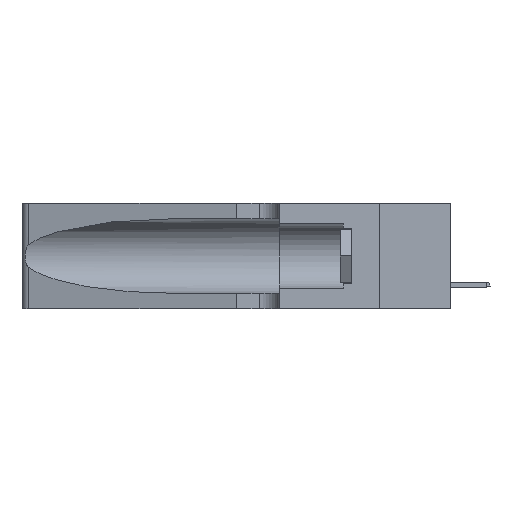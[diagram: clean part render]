
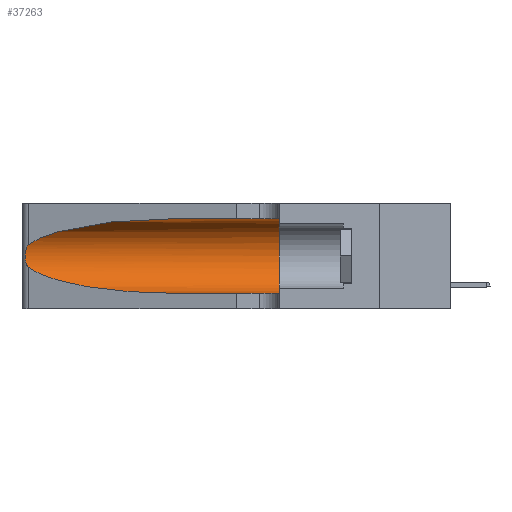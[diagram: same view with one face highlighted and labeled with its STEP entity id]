
A CAD part, left-side view. The second image highlights one B-rep face of the part: STEP entity #37263.
In plain terms, the highlighted cylindrical face has radius 3.308 mm (diameter 6.617 mm), a partial arc.
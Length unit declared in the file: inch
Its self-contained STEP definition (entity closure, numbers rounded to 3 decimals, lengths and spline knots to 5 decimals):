
#66 = CARTESIAN_POINT ( 'NONE',  ( 0.25787, 1.23484, 0.2124 ) ) ;
#715 = EDGE_CURVE ( 'NONE', #21930, #15753, #25304, .T. ) ;
#826 = EDGE_CURVE ( 'NONE', #28318, #10682, #22573, .T. ) ;
#1130 = VECTOR ( 'NONE', #39923, 39.37008 ) ;
#2950 = ORIENTED_EDGE ( 'NONE', *, *, #826, .F. ) ;
#2981 = CARTESIAN_POINT ( 'NONE',  ( 0.25639, 1.23186, 0.15144 ) ) ;
#3543 = CARTESIAN_POINT ( 'NONE',  ( 0.1305, 0.72297, 0.31525 ) ) ;
#3771 = VECTOR ( 'NONE', #42507, 39.37008 ) ;
#5016 = CARTESIAN_POINT ( 'NONE',  ( 0.1305, 0.35, 0.185 ) ) ;
#5486 = CARTESIAN_POINT ( 'NONE',  ( 0.1305, 0.72297, 0.05475 ) ) ;
#5630 =( BOUNDED_CURVE ( )  B_SPLINE_CURVE ( 3, ( #8468, #12322, #44951, #23143 ),
 .UNSPECIFIED., .F., .F. ) 
 B_SPLINE_CURVE_WITH_KNOTS ( ( 4, 4 ),
 ( 1.5708, 2.84003 ),
 .UNSPECIFIED. ) 
 CURVE ( )  GEOMETRIC_REPRESENTATION_ITEM ( )  RATIONAL_B_SPLINE_CURVE ( ( 1., 0.87, 0.87, 1. ) ) 
 REPRESENTATION_ITEM ( '' )  );
#7513 = CARTESIAN_POINT ( 'NONE',  ( 0.25789, 1.23486, 0.15765 ) ) ;
#8029 = B_SPLINE_CURVE_WITH_KNOTS ( 'NONE', 3,
 ( #18340, #46891, #32990, #66, #24863, #43992, #11125, #25817, #40397, #35882, #7513, #2981, #17635, #32294 ),
 .UNSPECIFIED., .F., .F.,
 ( 4, 2, 2, 2, 2, 2, 4 ),
 ( 0., 0.00027, 0.00053, 0.00107, 0.0016, 0.00187, 0.00214 ),
 .UNSPECIFIED. ) ;
#8468 = CARTESIAN_POINT ( 'NONE',  ( 0.1305, 0.72297, 0.31525 ) ) ;
#10322 = EDGE_CURVE ( 'NONE', #15753, #10682, #43202, .T. ) ;
#10682 = VERTEX_POINT ( 'NONE', #45807 ) ;
#11125 = CARTESIAN_POINT ( 'NONE',  ( 0.26075, 1.23896, 0.19203 ) ) ;
#12322 = CARTESIAN_POINT ( 'NONE',  ( 0.18966, 0.96281, 0.31525 ) ) ;
#12377 = ORIENTED_EDGE ( 'NONE', *, *, #33745, .T. ) ;
#12836 = CARTESIAN_POINT ( 'NONE',  ( 0.25487, 1.22718, 0.22369 ) ) ;
#14775 = CYLINDRICAL_SURFACE ( 'NONE', #37907, 0.13025 ) ;
#15117 = CARTESIAN_POINT ( 'NONE',  ( 0.2373, 1.15595, 0.08982 ) ) ;
#15423 = CARTESIAN_POINT ( 'NONE',  ( 0.1305, 0.72297, 0.05475 ) ) ;
#15638 = AXIS2_PLACEMENT_3D ( 'NONE', #5016, #19664, #34548 ) ;
#15753 = VERTEX_POINT ( 'NONE', #15423 ) ;
#16855 = EDGE_CURVE ( 'NONE', #20490, #42874, #5630, .T. ) ;
#17158 = ORIENTED_EDGE ( 'NONE', *, *, #715, .T. ) ;
#17635 = CARTESIAN_POINT ( 'NONE',  ( 0.25555, 1.22993, 0.14849 ) ) ;
#18340 = CARTESIAN_POINT ( 'NONE',  ( 0.25487, 1.22718, 0.22369 ) ) ;
#19155 = ORIENTED_EDGE ( 'NONE', *, *, #16855, .T. ) ;
#19664 = DIRECTION ( 'NONE',  ( 0., 1., 0. ) ) ;
#20490 = VERTEX_POINT ( 'NONE', #3543 ) ;
#21848 = CARTESIAN_POINT ( 'NONE',  ( 0.1305, 0.35, 0.31525 ) ) ;
#21930 = VERTEX_POINT ( 'NONE', #39190 ) ;
#22573 = CIRCLE ( 'NONE', #15638, 0.13025 ) ;
#22710 = CARTESIAN_POINT ( 'NONE',  ( 0.1305, 1.61858, 0.185 ) ) ;
#23143 = CARTESIAN_POINT ( 'NONE',  ( 0.25487, 1.22718, 0.22369 ) ) ;
#24863 = CARTESIAN_POINT ( 'NONE',  ( 0.25854, 1.2359, 0.20912 ) ) ;
#25304 =( BOUNDED_CURVE ( )  B_SPLINE_CURVE ( 3, ( #36257, #15117, #41716, #5486 ),
 .UNSPECIFIED., .F., .F. ) 
 B_SPLINE_CURVE_WITH_KNOTS ( ( 4, 4 ),
 ( 3.44316, 4.71239 ),
 .UNSPECIFIED. ) 
 CURVE ( )  GEOMETRIC_REPRESENTATION_ITEM ( )  RATIONAL_B_SPLINE_CURVE ( ( 1., 0.87, 0.87, 1. ) ) 
 REPRESENTATION_ITEM ( '' )  );
#25817 = CARTESIAN_POINT ( 'NONE',  ( 0.26075, 1.23896, 0.178 ) ) ;
#27987 = LINE ( 'NONE', #37043, #1130 ) ;
#28318 = VERTEX_POINT ( 'NONE', #21848 ) ;
#32294 = CARTESIAN_POINT ( 'NONE',  ( 0.25487, 1.22718, 0.14631 ) ) ;
#32990 = CARTESIAN_POINT ( 'NONE',  ( 0.25639, 1.23184, 0.21858 ) ) ;
#33269 = DIRECTION ( 'NONE',  ( 0., 0., -1. ) ) ;
#33745 = EDGE_CURVE ( 'NONE', #42874, #21930, #8029, .T. ) ;
#33747 = DIRECTION ( 'NONE',  ( 0., -1., 0. ) ) ;
#34548 = DIRECTION ( 'NONE',  ( 0., 0., 1. ) ) ;
#35882 = CARTESIAN_POINT ( 'NONE',  ( 0.25856, 1.23593, 0.16098 ) ) ;
#36257 = CARTESIAN_POINT ( 'NONE',  ( 0.25487, 1.22718, 0.14631 ) ) ;
#36394 = FACE_OUTER_BOUND ( 'NONE', #40631, .T. ) ;
#37043 = CARTESIAN_POINT ( 'NONE',  ( 0.1305, 1.61858, 0.31525 ) ) ;
#37263 = ADVANCED_FACE ( 'NONE', ( #36394 ), #14775, .F. ) ;
#37633 = EDGE_CURVE ( 'NONE', #20490, #28318, #27987, .T. ) ;
#37672 = ORIENTED_EDGE ( 'NONE', *, *, #37633, .F. ) ;
#37907 = AXIS2_PLACEMENT_3D ( 'NONE', #22710, #33747, #33269 ) ;
#39190 = CARTESIAN_POINT ( 'NONE',  ( 0.25487, 1.22718, 0.14631 ) ) ;
#39923 = DIRECTION ( 'NONE',  ( 0., -1., 0. ) ) ;
#40397 = CARTESIAN_POINT ( 'NONE',  ( 0.26017, 1.23833, 0.17102 ) ) ;
#40631 = EDGE_LOOP ( 'NONE', ( #19155, #12377, #17158, #44356, #2950, #37672 ) ) ;
#41716 = CARTESIAN_POINT ( 'NONE',  ( 0.18966, 0.96281, 0.05475 ) ) ;
#42507 = DIRECTION ( 'NONE',  ( 0., -1., 0. ) ) ;
#42874 = VERTEX_POINT ( 'NONE', #12836 ) ;
#43202 = LINE ( 'NONE', #46101, #3771 ) ;
#43992 = CARTESIAN_POINT ( 'NONE',  ( 0.26018, 1.23835, 0.19895 ) ) ;
#44356 = ORIENTED_EDGE ( 'NONE', *, *, #10322, .T. ) ;
#44951 = CARTESIAN_POINT ( 'NONE',  ( 0.2373, 1.15595, 0.28018 ) ) ;
#45807 = CARTESIAN_POINT ( 'NONE',  ( 0.1305, 0.35, 0.05475 ) ) ;
#46101 = CARTESIAN_POINT ( 'NONE',  ( 0.1305, 1.61858, 0.05475 ) ) ;
#46891 = CARTESIAN_POINT ( 'NONE',  ( 0.25555, 1.22994, 0.2215 ) ) ;
